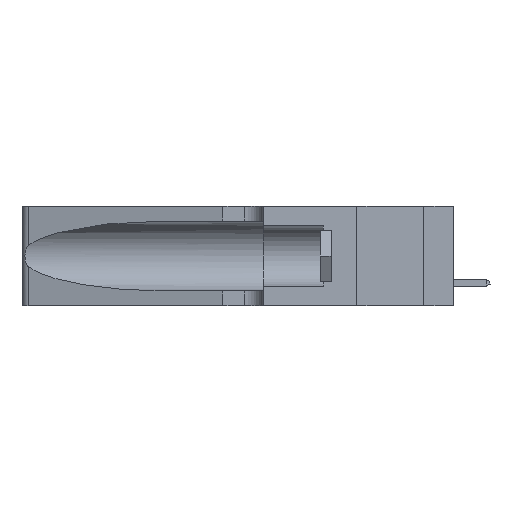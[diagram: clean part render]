
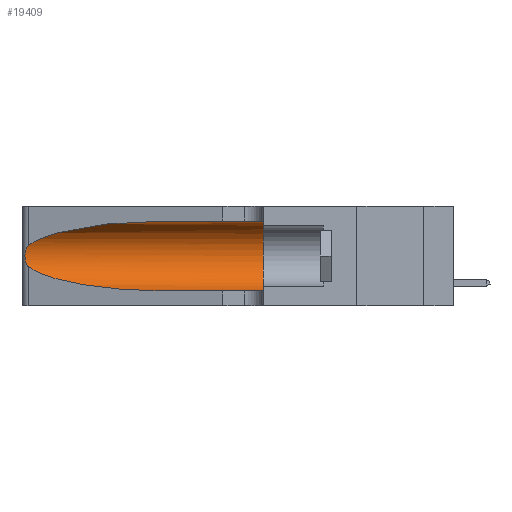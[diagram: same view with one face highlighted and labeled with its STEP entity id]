
A CAD part, left-side view. The second image highlights one B-rep face of the part: STEP entity #19409.
In plain terms, the highlighted cylindrical face has radius 3.308 mm (diameter 6.617 mm), a partial arc.
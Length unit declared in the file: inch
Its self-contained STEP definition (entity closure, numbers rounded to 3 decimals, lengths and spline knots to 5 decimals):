
#544 = CARTESIAN_POINT ( 'NONE',  ( 0.25487, 1.22718, 0.22369 ) ) ;
#1254 = DIRECTION ( 'NONE',  ( 0., 0., -1. ) ) ;
#1257 = ORIENTED_EDGE ( 'NONE', *, *, #13048, .T. ) ;
#1620 = CARTESIAN_POINT ( 'NONE',  ( 0.1305, 0.72297, 0.05475 ) ) ;
#2047 = CARTESIAN_POINT ( 'NONE',  ( 0.18966, 0.96281, 0.31525 ) ) ;
#3494 =( BOUNDED_CURVE ( )  B_SPLINE_CURVE ( 3, ( #6056, #2047, #8462, #16783 ),
 .UNSPECIFIED., .F., .F. ) 
 B_SPLINE_CURVE_WITH_KNOTS ( ( 4, 4 ),
 ( 1.5708, 2.84003 ),
 .UNSPECIFIED. ) 
 CURVE ( )  GEOMETRIC_REPRESENTATION_ITEM ( )  RATIONAL_B_SPLINE_CURVE ( ( 1., 0.87, 0.87, 1. ) ) 
 REPRESENTATION_ITEM ( '' )  );
#3527 = CARTESIAN_POINT ( 'NONE',  ( 0.1305, 0.35, 0.31525 ) ) ;
#3770 = LINE ( 'NONE', #15083, #8212 ) ;
#4024 = CIRCLE ( 'NONE', #25712, 0.13025 ) ;
#4922 = VECTOR ( 'NONE', #5436, 39.37008 ) ;
#4961 = B_SPLINE_CURVE_WITH_KNOTS ( 'NONE', 3,
 ( #544, #11997, #9678, #5639, #17993, #11829, #18430, #16435, #24720, #20472, #10283, #18267, #18174, #14216 ),
 .UNSPECIFIED., .F., .F.,
 ( 4, 2, 2, 2, 2, 2, 4 ),
 ( 0., 0.00027, 0.00053, 0.00107, 0.0016, 0.00187, 0.00214 ),
 .UNSPECIFIED. ) ;
#5436 = DIRECTION ( 'NONE',  ( 0., -1., 0. ) ) ;
#5639 = CARTESIAN_POINT ( 'NONE',  ( 0.25787, 1.23484, 0.2124 ) ) ;
#5865 = CARTESIAN_POINT ( 'NONE',  ( 0.1305, 0.72297, 0.05475 ) ) ;
#6056 = CARTESIAN_POINT ( 'NONE',  ( 0.1305, 0.72297, 0.31525 ) ) ;
#6108 = CYLINDRICAL_SURFACE ( 'NONE', #20807, 0.13025 ) ;
#6205 = DIRECTION ( 'NONE',  ( 0., -1., 0. ) ) ;
#6848 = EDGE_CURVE ( 'NONE', #7444, #7175, #4024, .T. ) ;
#7175 = VERTEX_POINT ( 'NONE', #10065 ) ;
#7444 = VERTEX_POINT ( 'NONE', #3527 ) ;
#7954 = ORIENTED_EDGE ( 'NONE', *, *, #13654, .T. ) ;
#8063 = CARTESIAN_POINT ( 'NONE',  ( 0.1305, 0.35, 0.185 ) ) ;
#8212 = VECTOR ( 'NONE', #25304, 39.37008 ) ;
#8257 = CARTESIAN_POINT ( 'NONE',  ( 0.1305, 1.61858, 0.31525 ) ) ;
#8343 = FACE_OUTER_BOUND ( 'NONE', #9703, .T. ) ;
#8462 = CARTESIAN_POINT ( 'NONE',  ( 0.2373, 1.15595, 0.28018 ) ) ;
#8878 = ORIENTED_EDGE ( 'NONE', *, *, #21487, .T. ) ;
#9678 = CARTESIAN_POINT ( 'NONE',  ( 0.25639, 1.23184, 0.21858 ) ) ;
#9703 = EDGE_LOOP ( 'NONE', ( #21379, #8878, #1257, #7954, #25484, #11672 ) ) ;
#9769 = CARTESIAN_POINT ( 'NONE',  ( 0.18966, 0.96281, 0.05475 ) ) ;
#10065 = CARTESIAN_POINT ( 'NONE',  ( 0.1305, 0.35, 0.05475 ) ) ;
#10067 = VERTEX_POINT ( 'NONE', #5865 ) ;
#10283 = CARTESIAN_POINT ( 'NONE',  ( 0.25789, 1.23486, 0.15765 ) ) ;
#10315 = DIRECTION ( 'NONE',  ( 0., 1., 0. ) ) ;
#11401 = EDGE_CURVE ( 'NONE', #22095, #24310, #3494, .T. ) ;
#11652 = CARTESIAN_POINT ( 'NONE',  ( 0.2373, 1.15595, 0.08982 ) ) ;
#11672 = ORIENTED_EDGE ( 'NONE', *, *, #16047, .F. ) ;
#11829 = CARTESIAN_POINT ( 'NONE',  ( 0.26018, 1.23835, 0.19895 ) ) ;
#11997 = CARTESIAN_POINT ( 'NONE',  ( 0.25555, 1.22994, 0.2215 ) ) ;
#12520 =( BOUNDED_CURVE ( )  B_SPLINE_CURVE ( 3, ( #13883, #11652, #9769, #1620 ),
 .UNSPECIFIED., .F., .F. ) 
 B_SPLINE_CURVE_WITH_KNOTS ( ( 4, 4 ),
 ( 3.44316, 4.71239 ),
 .UNSPECIFIED. ) 
 CURVE ( )  GEOMETRIC_REPRESENTATION_ITEM ( )  RATIONAL_B_SPLINE_CURVE ( ( 1., 0.87, 0.87, 1. ) ) 
 REPRESENTATION_ITEM ( '' )  );
#13048 = EDGE_CURVE ( 'NONE', #21970, #10067, #12520, .T. ) ;
#13654 = EDGE_CURVE ( 'NONE', #10067, #7175, #3770, .T. ) ;
#13883 = CARTESIAN_POINT ( 'NONE',  ( 0.25487, 1.22718, 0.14631 ) ) ;
#14216 = CARTESIAN_POINT ( 'NONE',  ( 0.25487, 1.22718, 0.14631 ) ) ;
#15083 = CARTESIAN_POINT ( 'NONE',  ( 0.1305, 1.61858, 0.05475 ) ) ;
#16047 = EDGE_CURVE ( 'NONE', #22095, #7444, #24819, .T. ) ;
#16435 = CARTESIAN_POINT ( 'NONE',  ( 0.26075, 1.23896, 0.178 ) ) ;
#16783 = CARTESIAN_POINT ( 'NONE',  ( 0.25487, 1.22718, 0.22369 ) ) ;
#17144 = CARTESIAN_POINT ( 'NONE',  ( 0.1305, 0.72297, 0.31525 ) ) ;
#17993 = CARTESIAN_POINT ( 'NONE',  ( 0.25854, 1.2359, 0.20912 ) ) ;
#18174 = CARTESIAN_POINT ( 'NONE',  ( 0.25555, 1.22993, 0.14849 ) ) ;
#18267 = CARTESIAN_POINT ( 'NONE',  ( 0.25639, 1.23186, 0.15144 ) ) ;
#18381 = DIRECTION ( 'NONE',  ( 0., 0., 1. ) ) ;
#18430 = CARTESIAN_POINT ( 'NONE',  ( 0.26075, 1.23896, 0.19203 ) ) ;
#19409 = ADVANCED_FACE ( 'NONE', ( #8343 ), #6108, .F. ) ;
#20472 = CARTESIAN_POINT ( 'NONE',  ( 0.25856, 1.23593, 0.16098 ) ) ;
#20807 = AXIS2_PLACEMENT_3D ( 'NONE', #24763, #6205, #1254 ) ;
#21379 = ORIENTED_EDGE ( 'NONE', *, *, #11401, .T. ) ;
#21487 = EDGE_CURVE ( 'NONE', #24310, #21970, #4961, .T. ) ;
#21970 = VERTEX_POINT ( 'NONE', #26154 ) ;
#22095 = VERTEX_POINT ( 'NONE', #17144 ) ;
#22939 = CARTESIAN_POINT ( 'NONE',  ( 0.25487, 1.22718, 0.22369 ) ) ;
#24310 = VERTEX_POINT ( 'NONE', #22939 ) ;
#24720 = CARTESIAN_POINT ( 'NONE',  ( 0.26017, 1.23833, 0.17102 ) ) ;
#24763 = CARTESIAN_POINT ( 'NONE',  ( 0.1305, 1.61858, 0.185 ) ) ;
#24819 = LINE ( 'NONE', #8257, #4922 ) ;
#25304 = DIRECTION ( 'NONE',  ( 0., -1., 0. ) ) ;
#25484 = ORIENTED_EDGE ( 'NONE', *, *, #6848, .F. ) ;
#25712 = AXIS2_PLACEMENT_3D ( 'NONE', #8063, #10315, #18381 ) ;
#26154 = CARTESIAN_POINT ( 'NONE',  ( 0.25487, 1.22718, 0.14631 ) ) ;
